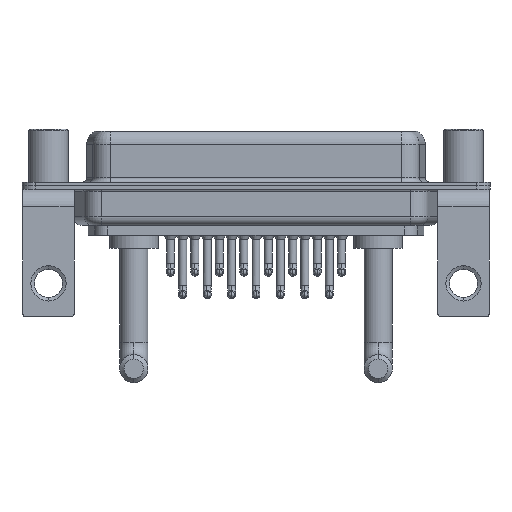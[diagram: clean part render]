
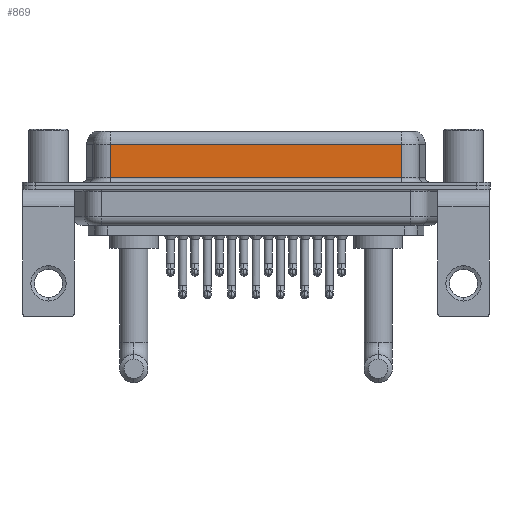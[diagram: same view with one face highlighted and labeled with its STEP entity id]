
A CAD part, front view. The second image highlights one B-rep face of the part: STEP entity #869.
In plain terms, the highlighted planar face has unit normal (0, -1, 0).
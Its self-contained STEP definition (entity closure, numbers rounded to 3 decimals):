
#382 = ORIENTED_EDGE ( 'NONE', *, *, #18394, .F. ) ;
#869 = ADVANCED_FACE ( 'NONE', ( #8160 ), #6375, .F. ) ;
#1088 = VECTOR ( 'NONE', #1163, 1000. ) ;
#1163 = DIRECTION ( 'NONE',  ( -1., 0., 0. ) ) ;
#1389 = ORIENTED_EDGE ( 'NONE', *, *, #22966, .T. ) ;
#1907 = ORIENTED_EDGE ( 'NONE', *, *, #9771, .T. ) ;
#2099 = CARTESIAN_POINT ( 'NONE',  ( 40.037, -3.95, 0.9 ) ) ;
#3158 = CARTESIAN_POINT ( 'NONE',  ( 40.037, -3.95, 0.9 ) ) ;
#4255 = CARTESIAN_POINT ( 'NONE',  ( 40.037, -3.95, 6.4 ) ) ;
#4494 = LINE ( 'NONE', #8056, #20832 ) ;
#5193 = CARTESIAN_POINT ( 'NONE',  ( 7.013, -3.95, 6.4 ) ) ;
#6375 = PLANE ( 'NONE',  #9657 ) ;
#6810 = DIRECTION ( 'NONE',  ( 1., 0., 0. ) ) ;
#8056 = CARTESIAN_POINT ( 'NONE',  ( 40.037, -3.95, 6.4 ) ) ;
#8160 = FACE_OUTER_BOUND ( 'NONE', #19911, .T. ) ;
#8256 = LINE ( 'NONE', #10134, #1088 ) ;
#8506 = LINE ( 'NONE', #5193, #18638 ) ;
#8586 = VERTEX_POINT ( 'NONE', #8855 ) ;
#8855 = CARTESIAN_POINT ( 'NONE',  ( 7.013, -3.95, 0.9 ) ) ;
#8915 = EDGE_CURVE ( 'NONE', #10504, #23221, #8256, .T. ) ;
#9657 = AXIS2_PLACEMENT_3D ( 'NONE', #4255, #13594, #19013 ) ;
#9771 = EDGE_CURVE ( 'NONE', #23221, #8586, #8506, .T. ) ;
#10134 = CARTESIAN_POINT ( 'NONE',  ( 40.037, -3.95, 4.65 ) ) ;
#10504 = VERTEX_POINT ( 'NONE', #18929 ) ;
#13594 = DIRECTION ( 'NONE',  ( 0., 1., 0. ) ) ;
#14594 = CARTESIAN_POINT ( 'NONE',  ( 7.013, -3.95, 4.65 ) ) ;
#15549 = LINE ( 'NONE', #3158, #23104 ) ;
#17481 = DIRECTION ( 'NONE',  ( 0., 0., -1. ) ) ;
#17949 = VERTEX_POINT ( 'NONE', #2099 ) ;
#18137 = DIRECTION ( 'NONE',  ( 0., 0., -1. ) ) ;
#18394 = EDGE_CURVE ( 'NONE', #10504, #17949, #4494, .T. ) ;
#18638 = VECTOR ( 'NONE', #18137, 1000. ) ;
#18929 = CARTESIAN_POINT ( 'NONE',  ( 40.037, -3.95, 4.65 ) ) ;
#19013 = DIRECTION ( 'NONE',  ( 0., 0., 1. ) ) ;
#19121 = ORIENTED_EDGE ( 'NONE', *, *, #8915, .T. ) ;
#19911 = EDGE_LOOP ( 'NONE', ( #382, #19121, #1907, #1389 ) ) ;
#20832 = VECTOR ( 'NONE', #17481, 1000. ) ;
#22966 = EDGE_CURVE ( 'NONE', #8586, #17949, #15549, .T. ) ;
#23104 = VECTOR ( 'NONE', #6810, 1000. ) ;
#23221 = VERTEX_POINT ( 'NONE', #14594 ) ;
